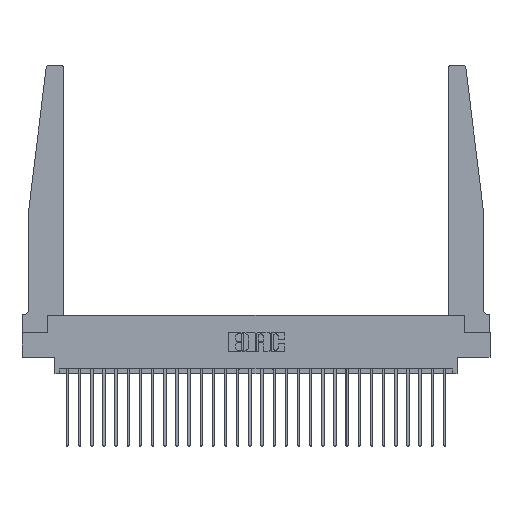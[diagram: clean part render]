
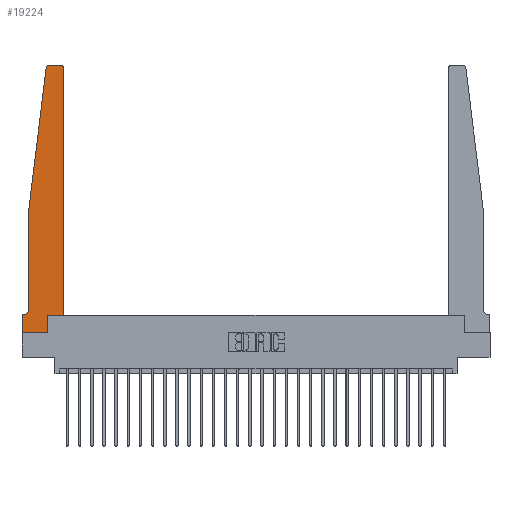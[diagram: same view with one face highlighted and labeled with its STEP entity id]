
A CAD part, top view. The second image highlights one B-rep face of the part: STEP entity #19224.
In plain terms, the highlighted planar face has unit normal (0, 0, 1).
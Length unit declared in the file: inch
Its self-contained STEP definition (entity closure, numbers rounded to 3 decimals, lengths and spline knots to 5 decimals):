
#358 = ORIENTED_EDGE ( 'NONE', *, *, #20026, .T. ) ;
#467 = ORIENTED_EDGE ( 'NONE', *, *, #24330, .T. ) ;
#490 = DIRECTION ( 'NONE',  ( 0., -1., 0. ) ) ;
#613 = VERTEX_POINT ( 'NONE', #24567 ) ;
#811 = VERTEX_POINT ( 'NONE', #26072 ) ;
#863 = AXIS2_PLACEMENT_3D ( 'NONE', #21619, #2489, #9863 ) ;
#1479 = LINE ( 'NONE', #3963, #14621 ) ;
#2377 = AXIS2_PLACEMENT_3D ( 'NONE', #13785, #6811, #13238 ) ;
#2489 = DIRECTION ( 'NONE',  ( 0., 0., 1. ) ) ;
#3267 = EDGE_LOOP ( 'NONE', ( #467, #16690, #7689, #11547, #19007, #23755, #15812, #358, #12655, #14020, #4505, #10604 ) ) ;
#3761 = CARTESIAN_POINT ( 'NONE',  ( 0.27653, 2.75, 0.37 ) ) ;
#3924 = LINE ( 'NONE', #17032, #22248 ) ;
#3963 = CARTESIAN_POINT ( 'NONE',  ( 0.065, 1.25, 0.37 ) ) ;
#4505 = ORIENTED_EDGE ( 'NONE', *, *, #19469, .T. ) ;
#4552 = EDGE_CURVE ( 'NONE', #21685, #24644, #3924, .T. ) ;
#4901 = DIRECTION ( 'NONE',  ( 1., 0., 0. ) ) ;
#5056 = VECTOR ( 'NONE', #490, 39.37008 ) ;
#5201 = EDGE_CURVE ( 'NONE', #21450, #811, #24512, .T. ) ;
#5692 = CARTESIAN_POINT ( 'NONE',  ( 0.24675, 2.72367, 0.37 ) ) ;
#6080 = EDGE_CURVE ( 'NONE', #27129, #22037, #1479, .T. ) ;
#6112 = CARTESIAN_POINT ( 'NONE',  ( 0.425, 0.18, 0.37 ) ) ;
#6811 = DIRECTION ( 'NONE',  ( 0., 0., 1. ) ) ;
#6847 = VECTOR ( 'NONE', #18710, 39.37008 ) ;
#7689 = ORIENTED_EDGE ( 'NONE', *, *, #6080, .T. ) ;
#8306 = DIRECTION ( 'NONE',  ( -1., 0., 0. ) ) ;
#8882 = CARTESIAN_POINT ( 'NONE',  ( 0., 0., 0.37 ) ) ;
#9628 = CARTESIAN_POINT ( 'NONE',  ( 0.015, 0.2375, 0.37 ) ) ;
#9767 = DIRECTION ( 'NONE',  ( -1., 0., 0. ) ) ;
#9863 = DIRECTION ( 'NONE',  ( 1., 0., 0. ) ) ;
#9909 = CARTESIAN_POINT ( 'NONE',  ( 0.2605, 0.18, 0.37 ) ) ;
#9988 = CARTESIAN_POINT ( 'NONE',  ( 0., 0., 0.37 ) ) ;
#10193 = LINE ( 'NONE', #9909, #6847 ) ;
#10409 = CARTESIAN_POINT ( 'NONE',  ( 0.065, 0.2375, 0.37 ) ) ;
#10604 = ORIENTED_EDGE ( 'NONE', *, *, #5201, .T. ) ;
#10738 = VECTOR ( 'NONE', #20677, 39.37008 ) ;
#10865 = EDGE_CURVE ( 'NONE', #22037, #14658, #13458, .T. ) ;
#11458 = EDGE_CURVE ( 'NONE', #14658, #14467, #27327, .T. ) ;
#11509 = DIRECTION ( 'NONE',  ( 1., 0., 0. ) ) ;
#11547 = ORIENTED_EDGE ( 'NONE', *, *, #10865, .T. ) ;
#11568 = VECTOR ( 'NONE', #11509, 39.37008 ) ;
#12137 = LINE ( 'NONE', #6112, #10738 ) ;
#12333 = LINE ( 'NONE', #9988, #22963 ) ;
#12441 = LINE ( 'NONE', #25314, #13959 ) ;
#12655 = ORIENTED_EDGE ( 'NONE', *, *, #24822, .T. ) ;
#13238 = DIRECTION ( 'NONE',  ( 1., 0., 0. ) ) ;
#13458 = LINE ( 'NONE', #15556, #5056 ) ;
#13785 = CARTESIAN_POINT ( 'NONE',  ( 0.27653, 2.72, 0.37 ) ) ;
#13959 = VECTOR ( 'NONE', #18471, 39.37008 ) ;
#13975 = VERTEX_POINT ( 'NONE', #15362 ) ;
#14020 = ORIENTED_EDGE ( 'NONE', *, *, #4552, .T. ) ;
#14046 = VERTEX_POINT ( 'NONE', #3761 ) ;
#14467 = VERTEX_POINT ( 'NONE', #26648 ) ;
#14621 = VECTOR ( 'NONE', #23106, 39.37008 ) ;
#14658 = VERTEX_POINT ( 'NONE', #10409 ) ;
#14714 = PLANE ( 'NONE',  #19218 ) ;
#14741 = EDGE_CURVE ( 'NONE', #14467, #613, #21041, .T. ) ;
#14868 = CARTESIAN_POINT ( 'NONE',  ( 0.065, 0.1875, 0.37 ) ) ;
#14992 = DIRECTION ( 'NONE',  ( 0., 0., 1. ) ) ;
#15272 = AXIS2_PLACEMENT_3D ( 'NONE', #9628, #26705, #9767 ) ;
#15362 = CARTESIAN_POINT ( 'NONE',  ( 0.2605, 0., 0.37 ) ) ;
#15523 = CARTESIAN_POINT ( 'NONE',  ( 0., 0.1875, 0.37 ) ) ;
#15556 = CARTESIAN_POINT ( 'NONE',  ( 0.065, 1.25, 0.37 ) ) ;
#15812 = ORIENTED_EDGE ( 'NONE', *, *, #25665, .T. ) ;
#16074 = CARTESIAN_POINT ( 'NONE',  ( 0.425, 0.18, 0.37 ) ) ;
#16147 = DIRECTION ( 'NONE',  ( 0., -1., 0. ) ) ;
#16690 = ORIENTED_EDGE ( 'NONE', *, *, #23754, .T. ) ;
#17032 = CARTESIAN_POINT ( 'NONE',  ( 0.425, 0.18, 0.37 ) ) ;
#17189 = VECTOR ( 'NONE', #8306, 39.37008 ) ;
#17264 = CARTESIAN_POINT ( 'NONE',  ( 0.425, 2.72, 0.37 ) ) ;
#17660 = CARTESIAN_POINT ( 'NONE',  ( 0.065, 1.25, 0.37 ) ) ;
#18471 = DIRECTION ( 'NONE',  ( -1., 0., 0. ) ) ;
#18710 = DIRECTION ( 'NONE',  ( 0., 1., 0. ) ) ;
#19007 = ORIENTED_EDGE ( 'NONE', *, *, #11458, .T. ) ;
#19084 = LINE ( 'NONE', #8882, #11568 ) ;
#19218 = AXIS2_PLACEMENT_3D ( 'NONE', #15523, #14992, #4901 ) ;
#19224 = ADVANCED_FACE ( 'NONE', ( #21020 ), #14714, .T. ) ;
#19469 = EDGE_CURVE ( 'NONE', #24644, #21450, #12137, .T. ) ;
#20026 = EDGE_CURVE ( 'NONE', #20143, #13975, #19084, .T. ) ;
#20143 = VERTEX_POINT ( 'NONE', #21738 ) ;
#20677 = DIRECTION ( 'NONE',  ( 0., 1., 0. ) ) ;
#21020 = FACE_OUTER_BOUND ( 'NONE', #3267, .T. ) ;
#21041 = LINE ( 'NONE', #14868, #17189 ) ;
#21373 = DIRECTION ( 'NONE',  ( 1., 0., 0. ) ) ;
#21450 = VERTEX_POINT ( 'NONE', #17264 ) ;
#21619 = CARTESIAN_POINT ( 'NONE',  ( 0.395, 2.72, 0.37 ) ) ;
#21685 = VERTEX_POINT ( 'NONE', #26504 ) ;
#21738 = CARTESIAN_POINT ( 'NONE',  ( 0., 0., 0.37 ) ) ;
#22037 = VERTEX_POINT ( 'NONE', #17660 ) ;
#22248 = VECTOR ( 'NONE', #21373, 39.37008 ) ;
#22963 = VECTOR ( 'NONE', #16147, 39.37008 ) ;
#23106 = DIRECTION ( 'NONE',  ( -0.122, -0.992, 0. ) ) ;
#23754 = EDGE_CURVE ( 'NONE', #14046, #27129, #27349, .T. ) ;
#23755 = ORIENTED_EDGE ( 'NONE', *, *, #14741, .T. ) ;
#24330 = EDGE_CURVE ( 'NONE', #811, #14046, #12441, .T. ) ;
#24512 = CIRCLE ( 'NONE', #863, 0.03 ) ;
#24567 = CARTESIAN_POINT ( 'NONE',  ( 0., 0.1875, 0.37 ) ) ;
#24644 = VERTEX_POINT ( 'NONE', #16074 ) ;
#24822 = EDGE_CURVE ( 'NONE', #13975, #21685, #10193, .T. ) ;
#25314 = CARTESIAN_POINT ( 'NONE',  ( 0.25, 2.75, 0.37 ) ) ;
#25665 = EDGE_CURVE ( 'NONE', #613, #20143, #12333, .T. ) ;
#26072 = CARTESIAN_POINT ( 'NONE',  ( 0.395, 2.75, 0.37 ) ) ;
#26504 = CARTESIAN_POINT ( 'NONE',  ( 0.2605, 0.18, 0.37 ) ) ;
#26648 = CARTESIAN_POINT ( 'NONE',  ( 0.015, 0.1875, 0.37 ) ) ;
#26705 = DIRECTION ( 'NONE',  ( 0., 0., -1. ) ) ;
#27129 = VERTEX_POINT ( 'NONE', #5692 ) ;
#27327 = CIRCLE ( 'NONE', #15272, 0.05 ) ;
#27349 = CIRCLE ( 'NONE', #2377, 0.03 ) ;
